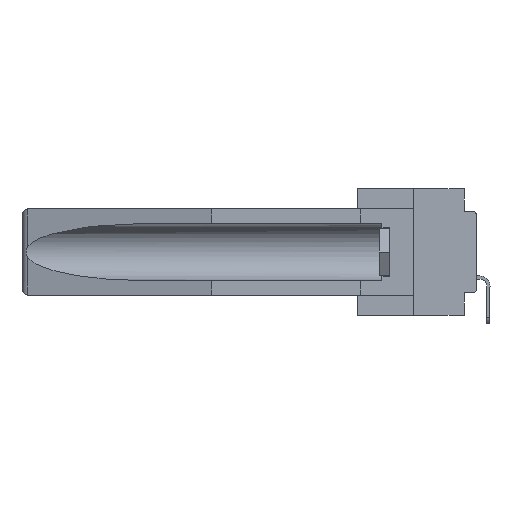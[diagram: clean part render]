
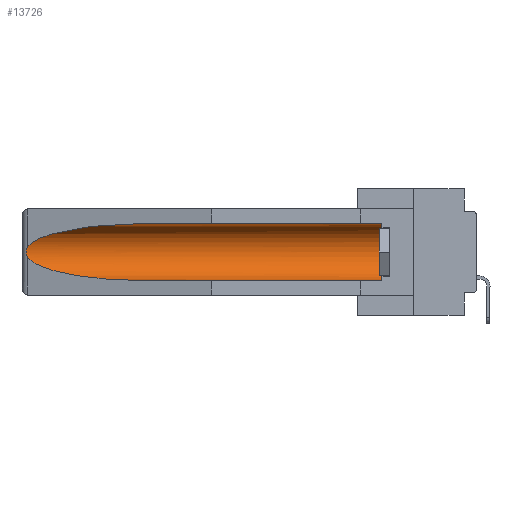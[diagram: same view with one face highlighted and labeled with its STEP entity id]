
A CAD part, left-side view. The second image highlights one B-rep face of the part: STEP entity #13726.
In plain terms, the highlighted cylindrical face has radius 2.857 mm (diameter 5.715 mm), a partial arc.
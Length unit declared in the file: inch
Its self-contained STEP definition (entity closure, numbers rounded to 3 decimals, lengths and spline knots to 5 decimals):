
#51 = CARTESIAN_POINT ( 'NONE',  ( 0.26537, 1.52718, -0.19328 ) ) ;
#284 = EDGE_CURVE ( 'NONE', #8151, #1099, #29889, .T. ) ;
#299 = ORIENTED_EDGE ( 'NONE', *, *, #599, .F. ) ;
#599 = EDGE_CURVE ( 'NONE', #2857, #15174, #23076, .T. ) ;
#931 = DIRECTION ( 'NONE',  ( 0., 1., 0. ) ) ;
#1099 = VERTEX_POINT ( 'NONE', #11320 ) ;
#1565 = ORIENTED_EDGE ( 'NONE', *, *, #12230, .T. ) ;
#2857 = VERTEX_POINT ( 'NONE', #23102 ) ;
#3195 = VERTEX_POINT ( 'NONE', #12756 ) ;
#5320 = CARTESIAN_POINT ( 'NONE',  ( 0.26537, 1.52718, -0.14972 ) ) ;
#5550 =( BOUNDED_CURVE ( )  B_SPLINE_CURVE ( 3, ( #29129, #9991, #17096, #5320 ),
 .UNSPECIFIED., .F., .F. ) 
 B_SPLINE_CURVE_WITH_KNOTS ( ( 4, 4 ),
 ( 4.71239, 6.08839 ),
 .UNSPECIFIED. ) 
 CURVE ( )  GEOMETRIC_REPRESENTATION_ITEM ( )  RATIONAL_B_SPLINE_CURVE ( ( 1., 0.848, 0.848, 1. ) ) 
 REPRESENTATION_ITEM ( '' )  );
#5634 = CARTESIAN_POINT ( 'NONE',  ( 0.26537, 1.52718, -0.14972 ) ) ;
#6104 = CARTESIAN_POINT ( 'NONE',  ( 0.2675, 1.53308, -0.16763 ) ) ;
#6425 = FACE_OUTER_BOUND ( 'NONE', #31081, .T. ) ;
#6524 = CARTESIAN_POINT ( 'NONE',  ( 0.2675, 1.53308, -0.17534 ) ) ;
#6782 = AXIS2_PLACEMENT_3D ( 'NONE', #15669, #931, #10787 ) ;
#8151 = VERTEX_POINT ( 'NONE', #5634 ) ;
#8197 = DIRECTION ( 'NONE',  ( 0., 0., 1. ) ) ;
#8308 = DIRECTION ( 'NONE',  ( 0., 1., 0. ) ) ;
#8426 = CARTESIAN_POINT ( 'NONE',  ( 0.155, -0.30754, -0.284 ) ) ;
#8857 =( BOUNDED_CURVE ( )  B_SPLINE_CURVE ( 3, ( #51, #18890, #21515, #19195 ),
 .UNSPECIFIED., .F., .F. ) 
 B_SPLINE_CURVE_WITH_KNOTS ( ( 4, 4 ),
 ( 0.1948, 1.5708 ),
 .UNSPECIFIED. ) 
 CURVE ( )  GEOMETRIC_REPRESENTATION_ITEM ( )  RATIONAL_B_SPLINE_CURVE ( ( 1., 0.848, 0.848, 1. ) ) 
 REPRESENTATION_ITEM ( '' )  );
#8968 = CARTESIAN_POINT ( 'NONE',  ( 0.26655, 1.53094, -0.18657 ) ) ;
#9805 = CIRCLE ( 'NONE', #14233, 0.1125 ) ;
#9970 = LINE ( 'NONE', #24500, #16326 ) ;
#9991 = CARTESIAN_POINT ( 'NONE',  ( 0.21114, 1.30732, -0.059 ) ) ;
#10074 = ORIENTED_EDGE ( 'NONE', *, *, #19260, .T. ) ;
#10169 = DIRECTION ( 'NONE',  ( 0., 1., 0. ) ) ;
#10787 = DIRECTION ( 'NONE',  ( 0., 0., 1. ) ) ;
#11097 = CARTESIAN_POINT ( 'NONE',  ( 0.26597, 1.52961, -0.15275 ) ) ;
#11200 = CARTESIAN_POINT ( 'NONE',  ( 0.26537, 1.52718, -0.19328 ) ) ;
#11320 = CARTESIAN_POINT ( 'NONE',  ( 0.26537, 1.52718, -0.19328 ) ) ;
#11712 = ORIENTED_EDGE ( 'NONE', *, *, #284, .T. ) ;
#12230 = EDGE_CURVE ( 'NONE', #24762, #8151, #5550, .T. ) ;
#12756 = CARTESIAN_POINT ( 'NONE',  ( 0.155, 0.126, -0.059 ) ) ;
#13726 = ADVANCED_FACE ( 'NONE', ( #6425 ), #29398, .F. ) ;
#14233 = AXIS2_PLACEMENT_3D ( 'NONE', #25195, #20141, #8197 ) ;
#14359 = EDGE_CURVE ( 'NONE', #2857, #3195, #9805, .T. ) ;
#14482 = CARTESIAN_POINT ( 'NONE',  ( 0.155, 1.07973, -0.059 ) ) ;
#15174 = VERTEX_POINT ( 'NONE', #21356 ) ;
#15669 = CARTESIAN_POINT ( 'NONE',  ( 0.155, -0.30754, -0.1715 ) ) ;
#16326 = VECTOR ( 'NONE', #10169, 39.37008 ) ;
#16694 = VECTOR ( 'NONE', #8308, 39.37008 ) ;
#17096 = CARTESIAN_POINT ( 'NONE',  ( 0.25451, 1.48313, -0.09465 ) ) ;
#18165 = EDGE_CURVE ( 'NONE', #3195, #24762, #9970, .T. ) ;
#18890 = CARTESIAN_POINT ( 'NONE',  ( 0.25451, 1.48313, -0.24835 ) ) ;
#19195 = CARTESIAN_POINT ( 'NONE',  ( 0.155, 1.07973, -0.284 ) ) ;
#19260 = EDGE_CURVE ( 'NONE', #1099, #15174, #8857, .T. ) ;
#20141 = DIRECTION ( 'NONE',  ( 0., -1., 0. ) ) ;
#20486 = CARTESIAN_POINT ( 'NONE',  ( 0.2673, 1.5327, -0.16383 ) ) ;
#21356 = CARTESIAN_POINT ( 'NONE',  ( 0.155, 1.07973, -0.284 ) ) ;
#21515 = CARTESIAN_POINT ( 'NONE',  ( 0.21114, 1.30732, -0.284 ) ) ;
#23076 = LINE ( 'NONE', #8426, #16694 ) ;
#23102 = CARTESIAN_POINT ( 'NONE',  ( 0.155, 0.126, -0.284 ) ) ;
#23316 = CARTESIAN_POINT ( 'NONE',  ( 0.26597, 1.5296, -0.19026 ) ) ;
#24500 = CARTESIAN_POINT ( 'NONE',  ( 0.155, -0.30754, -0.059 ) ) ;
#24762 = VERTEX_POINT ( 'NONE', #14482 ) ;
#25195 = CARTESIAN_POINT ( 'NONE',  ( 0.155, 0.126, -0.1715 ) ) ;
#25852 = CARTESIAN_POINT ( 'NONE',  ( 0.2673, 1.53269, -0.17917 ) ) ;
#27667 = CARTESIAN_POINT ( 'NONE',  ( 0.26537, 1.52718, -0.14972 ) ) ;
#27872 = CARTESIAN_POINT ( 'NONE',  ( 0.26654, 1.53092, -0.15636 ) ) ;
#28469 = ORIENTED_EDGE ( 'NONE', *, *, #14359, .T. ) ;
#29129 = CARTESIAN_POINT ( 'NONE',  ( 0.155, 1.07973, -0.059 ) ) ;
#29398 = CYLINDRICAL_SURFACE ( 'NONE', #6782, 0.1125 ) ;
#29889 = B_SPLINE_CURVE_WITH_KNOTS ( 'NONE', 3,
 ( #27667, #11097, #27872, #20486, #6104, #6524, #25852, #8968, #23316, #11200 ),
 .UNSPECIFIED., .F., .F.,
 ( 4, 2, 2, 2, 4 ),
 ( 0., 0.00029, 0.00058, 0.00087, 0.00117 ),
 .UNSPECIFIED. ) ;
#31001 = ORIENTED_EDGE ( 'NONE', *, *, #18165, .T. ) ;
#31081 = EDGE_LOOP ( 'NONE', ( #1565, #11712, #10074, #299, #28469, #31001 ) ) ;
